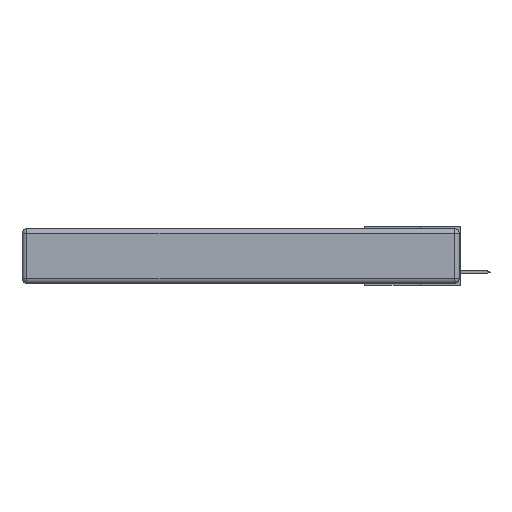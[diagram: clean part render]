
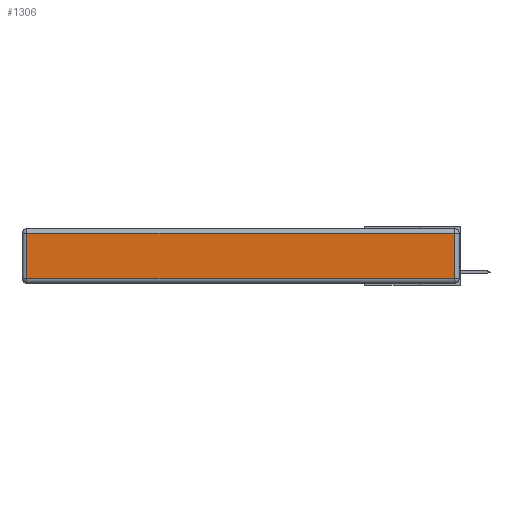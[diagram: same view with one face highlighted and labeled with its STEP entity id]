
A CAD part, left-side view. The second image highlights one B-rep face of the part: STEP entity #1306.
In plain terms, the highlighted planar face has unit normal (-1, 0, 0).
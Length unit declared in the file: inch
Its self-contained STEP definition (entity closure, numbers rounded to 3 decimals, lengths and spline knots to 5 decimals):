
#490 = DIRECTION ( 'NONE',  ( 0., -1., 0. ) ) ;
#556 = CARTESIAN_POINT ( 'NONE',  ( 0., 0., -0.343 ) ) ;
#813 = DIRECTION ( 'NONE',  ( 0., 1., 0. ) ) ;
#860 = LINE ( 'NONE', #1300, #10537 ) ;
#1300 = CARTESIAN_POINT ( 'NONE',  ( 0., 0., -0.313 ) ) ;
#1306 = ADVANCED_FACE ( 'NONE', ( #10663 ), #8092, .T. ) ;
#1461 = CARTESIAN_POINT ( 'NONE',  ( 0., 2.72, -0.343 ) ) ;
#1664 = LINE ( 'NONE', #3408, #12067 ) ;
#1669 = VERTEX_POINT ( 'NONE', #11030 ) ;
#3173 = ORIENTED_EDGE ( 'NONE', *, *, #5475, .T. ) ;
#3408 = CARTESIAN_POINT ( 'NONE',  ( 0., 2.75, -0.03 ) ) ;
#4284 = ORIENTED_EDGE ( 'NONE', *, *, #11466, .T. ) ;
#4343 = VECTOR ( 'NONE', #14072, 39.37008 ) ;
#4358 = DIRECTION ( 'NONE',  ( -1., 0., 0. ) ) ;
#4896 = VERTEX_POINT ( 'NONE', #10625 ) ;
#5195 = VERTEX_POINT ( 'NONE', #7691 ) ;
#5475 = EDGE_CURVE ( 'NONE', #1669, #4896, #860, .T. ) ;
#5940 = ORIENTED_EDGE ( 'NONE', *, *, #7526, .T. ) ;
#6756 = ORIENTED_EDGE ( 'NONE', *, *, #15441, .T. ) ;
#7526 = EDGE_CURVE ( 'NONE', #4896, #10737, #10570, .T. ) ;
#7691 = CARTESIAN_POINT ( 'NONE',  ( 0., 2.72, -0.03 ) ) ;
#7998 = VECTOR ( 'NONE', #13740, 39.37008 ) ;
#8092 = PLANE ( 'NONE',  #12277 ) ;
#9083 = EDGE_LOOP ( 'NONE', ( #3173, #5940, #6756, #4284 ) ) ;
#10008 = CARTESIAN_POINT ( 'NONE',  ( 0., 0.03, -0.343 ) ) ;
#10537 = VECTOR ( 'NONE', #490, 39.37008 ) ;
#10570 = LINE ( 'NONE', #10008, #7998 ) ;
#10625 = CARTESIAN_POINT ( 'NONE',  ( 0., 0.03, -0.313 ) ) ;
#10663 = FACE_OUTER_BOUND ( 'NONE', #9083, .T. ) ;
#10737 = VERTEX_POINT ( 'NONE', #15580 ) ;
#11030 = CARTESIAN_POINT ( 'NONE',  ( 0., 2.72, -0.313 ) ) ;
#11466 = EDGE_CURVE ( 'NONE', #5195, #1669, #11615, .T. ) ;
#11615 = LINE ( 'NONE', #1461, #4343 ) ;
#12067 = VECTOR ( 'NONE', #813, 39.37008 ) ;
#12277 = AXIS2_PLACEMENT_3D ( 'NONE', #556, #4358, #14457 ) ;
#13740 = DIRECTION ( 'NONE',  ( 0., 0., 1. ) ) ;
#14072 = DIRECTION ( 'NONE',  ( 0., 0., -1. ) ) ;
#14457 = DIRECTION ( 'NONE',  ( 0., 0., 1. ) ) ;
#15441 = EDGE_CURVE ( 'NONE', #10737, #5195, #1664, .T. ) ;
#15580 = CARTESIAN_POINT ( 'NONE',  ( 0., 0.03, -0.03 ) ) ;
